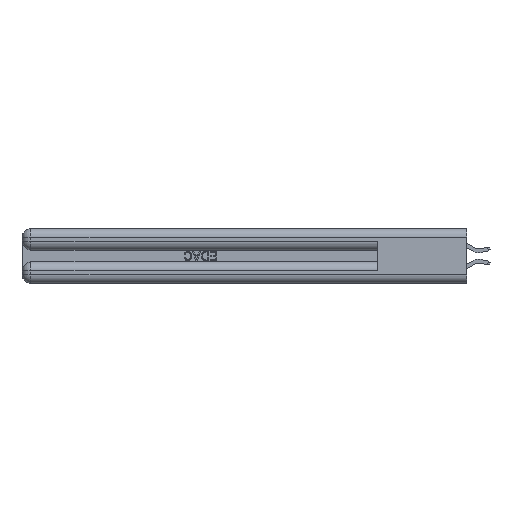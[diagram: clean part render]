
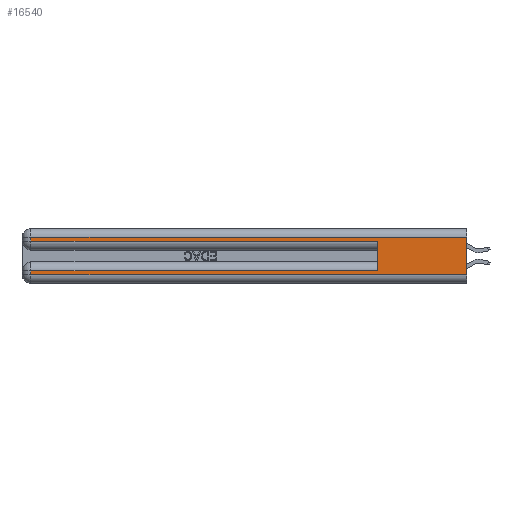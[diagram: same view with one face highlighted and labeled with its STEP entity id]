
A CAD part, left-side view. The second image highlights one B-rep face of the part: STEP entity #16540.
In plain terms, the highlighted planar face has unit normal (-1, 0, 0).
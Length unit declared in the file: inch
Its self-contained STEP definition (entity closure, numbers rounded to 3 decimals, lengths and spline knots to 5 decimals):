
#197 = EDGE_LOOP ( 'NONE', ( #18756, #33379, #35670, #15349, #27345, #12348, #12437, #24372 ) ) ;
#487 = EDGE_CURVE ( 'NONE', #25838, #37771, #37270, .T. ) ;
#649 = VECTOR ( 'NONE', #12497, 39.37008 ) ;
#795 = VERTEX_POINT ( 'NONE', #11955 ) ;
#1469 = VECTOR ( 'NONE', #25466, 39.37008 ) ;
#1845 = VECTOR ( 'NONE', #41381, 39.37008 ) ;
#2932 = LINE ( 'NONE', #2971, #1469 ) ;
#2971 = CARTESIAN_POINT ( 'NONE',  ( 0., 0.6, 0.145 ) ) ;
#3093 = CARTESIAN_POINT ( 'NONE',  ( 0., 0., 0.285 ) ) ;
#4457 = EDGE_CURVE ( 'NONE', #16725, #25838, #16438, .T. ) ;
#4743 = CARTESIAN_POINT ( 'NONE',  ( 0., 0., 0.06 ) ) ;
#5180 = PLANE ( 'NONE',  #23210 ) ;
#6344 = LINE ( 'NONE', #7033, #31473 ) ;
#6813 = DIRECTION ( 'NONE',  ( 0., 1., 0. ) ) ;
#7033 = CARTESIAN_POINT ( 'NONE',  ( 0., 0., 0.31 ) ) ;
#8792 = CARTESIAN_POINT ( 'NONE',  ( 0., 0., 0.37 ) ) ;
#10826 = CARTESIAN_POINT ( 'NONE',  ( 0., 0., 0.06 ) ) ;
#11178 = VERTEX_POINT ( 'NONE', #23234 ) ;
#11484 = CARTESIAN_POINT ( 'NONE',  ( 0., 2.94, 0.285 ) ) ;
#11955 = CARTESIAN_POINT ( 'NONE',  ( 0., 0.6, 0.085 ) ) ;
#12348 = ORIENTED_EDGE ( 'NONE', *, *, #25257, .T. ) ;
#12376 = LINE ( 'NONE', #18224, #34448 ) ;
#12437 = ORIENTED_EDGE ( 'NONE', *, *, #4457, .T. ) ;
#12497 = DIRECTION ( 'NONE',  ( 0., 0., -1. ) ) ;
#12903 = EDGE_CURVE ( 'NONE', #15292, #39547, #6344, .T. ) ;
#13209 = EDGE_CURVE ( 'NONE', #39547, #24938, #12376, .T. ) ;
#14677 = VECTOR ( 'NONE', #27522, 39.37008 ) ;
#15292 = VERTEX_POINT ( 'NONE', #37368 ) ;
#15349 = ORIENTED_EDGE ( 'NONE', *, *, #28994, .T. ) ;
#16438 = LINE ( 'NONE', #34872, #1845 ) ;
#16540 = ADVANCED_FACE ( 'NONE', ( #27690 ), #5180, .F. ) ;
#16725 = VERTEX_POINT ( 'NONE', #41376 ) ;
#18224 = CARTESIAN_POINT ( 'NONE',  ( 0., 2.94, 0.37 ) ) ;
#18371 = DIRECTION ( 'NONE',  ( 0., 0., -1. ) ) ;
#18526 = CARTESIAN_POINT ( 'NONE',  ( 0., 0., 0.37 ) ) ;
#18756 = ORIENTED_EDGE ( 'NONE', *, *, #24518, .F. ) ;
#19958 = DIRECTION ( 'NONE',  ( 0., 1., 0. ) ) ;
#20703 = CARTESIAN_POINT ( 'NONE',  ( 0., 2.94, 0.31 ) ) ;
#21743 = VECTOR ( 'NONE', #25860, 39.37008 ) ;
#23210 = AXIS2_PLACEMENT_3D ( 'NONE', #8792, #24724, #34597 ) ;
#23234 = CARTESIAN_POINT ( 'NONE',  ( 0., 0.6, 0.285 ) ) ;
#24372 = ORIENTED_EDGE ( 'NONE', *, *, #487, .T. ) ;
#24518 = EDGE_CURVE ( 'NONE', #15292, #37771, #41343, .T. ) ;
#24724 = DIRECTION ( 'NONE',  ( 1., 0., 0. ) ) ;
#24938 = VERTEX_POINT ( 'NONE', #11484 ) ;
#25257 = EDGE_CURVE ( 'NONE', #795, #16725, #36274, .T. ) ;
#25466 = DIRECTION ( 'NONE',  ( 0., 0., 1. ) ) ;
#25838 = VERTEX_POINT ( 'NONE', #26447 ) ;
#25860 = DIRECTION ( 'NONE',  ( 0., -1., 0. ) ) ;
#26447 = CARTESIAN_POINT ( 'NONE',  ( 0., 2.94, 0.06 ) ) ;
#26862 = EDGE_CURVE ( 'NONE', #795, #11178, #2932, .T. ) ;
#27345 = ORIENTED_EDGE ( 'NONE', *, *, #26862, .F. ) ;
#27522 = DIRECTION ( 'NONE',  ( 0., -1., 0. ) ) ;
#27690 = FACE_OUTER_BOUND ( 'NONE', #197, .T. ) ;
#28994 = EDGE_CURVE ( 'NONE', #24938, #11178, #34691, .T. ) ;
#31473 = VECTOR ( 'NONE', #19958, 39.37008 ) ;
#33379 = ORIENTED_EDGE ( 'NONE', *, *, #12903, .T. ) ;
#34448 = VECTOR ( 'NONE', #18371, 39.37008 ) ;
#34597 = DIRECTION ( 'NONE',  ( 0., 0., -1. ) ) ;
#34691 = LINE ( 'NONE', #3093, #21743 ) ;
#34872 = CARTESIAN_POINT ( 'NONE',  ( 0., 2.94, 0.37 ) ) ;
#35670 = ORIENTED_EDGE ( 'NONE', *, *, #13209, .T. ) ;
#35868 = CARTESIAN_POINT ( 'NONE',  ( 0., 0., 0.085 ) ) ;
#36274 = LINE ( 'NONE', #35868, #40783 ) ;
#37270 = LINE ( 'NONE', #10826, #14677 ) ;
#37368 = CARTESIAN_POINT ( 'NONE',  ( 0., 0., 0.31 ) ) ;
#37771 = VERTEX_POINT ( 'NONE', #4743 ) ;
#39547 = VERTEX_POINT ( 'NONE', #20703 ) ;
#40783 = VECTOR ( 'NONE', #6813, 39.37008 ) ;
#41343 = LINE ( 'NONE', #18526, #649 ) ;
#41376 = CARTESIAN_POINT ( 'NONE',  ( 0., 2.94, 0.085 ) ) ;
#41381 = DIRECTION ( 'NONE',  ( 0., 0., -1. ) ) ;
